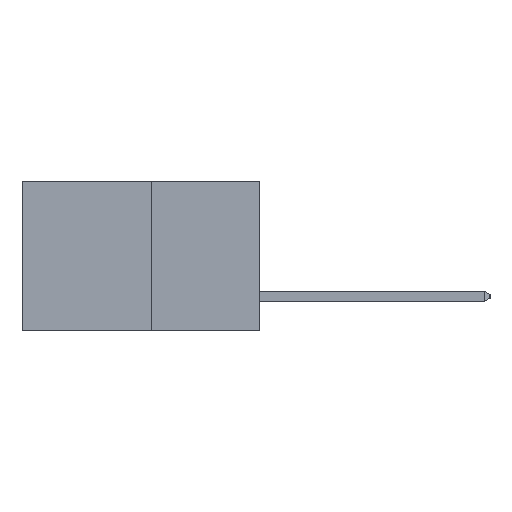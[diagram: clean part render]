
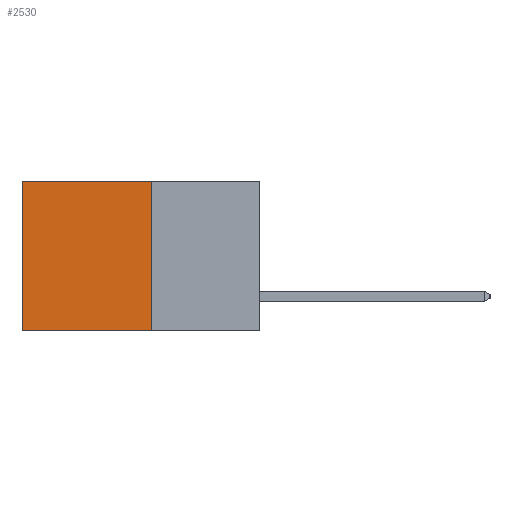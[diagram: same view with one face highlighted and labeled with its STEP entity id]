
A CAD part, left-side view. The second image highlights one B-rep face of the part: STEP entity #2530.
In plain terms, the highlighted planar face has unit normal (-1, 0, 0).
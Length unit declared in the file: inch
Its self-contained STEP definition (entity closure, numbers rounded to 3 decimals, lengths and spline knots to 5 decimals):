
#269 = EDGE_CURVE ( 'NONE', #4566, #11346, #6845, .T. ) ;
#826 = ORIENTED_EDGE ( 'NONE', *, *, #269, .T. ) ;
#2530 = ADVANCED_FACE ( 'NONE', ( #14349 ), #8832, .F. ) ;
#2600 = CARTESIAN_POINT ( 'NONE',  ( 0.277, 0.27, -0.37 ) ) ;
#3356 = EDGE_CURVE ( 'NONE', #13650, #11346, #5450, .T. ) ;
#4566 = VERTEX_POINT ( 'NONE', #12844 ) ;
#5028 = ORIENTED_EDGE ( 'NONE', *, *, #11836, .F. ) ;
#5037 = VECTOR ( 'NONE', #8416, 39.37008 ) ;
#5208 = DIRECTION ( 'NONE',  ( 0., 0., -1. ) ) ;
#5450 = LINE ( 'NONE', #8493, #5037 ) ;
#5720 = EDGE_CURVE ( 'NONE', #11275, #4566, #12967, .T. ) ;
#6845 = LINE ( 'NONE', #14623, #16168 ) ;
#8416 = DIRECTION ( 'NONE',  ( 0., 1., 0. ) ) ;
#8447 = DIRECTION ( 'NONE',  ( 0., 0., -1. ) ) ;
#8493 = CARTESIAN_POINT ( 'NONE',  ( 0.277, 0.27, -0.37 ) ) ;
#8512 = DIRECTION ( 'NONE',  ( 1., 0., 0. ) ) ;
#8688 = CARTESIAN_POINT ( 'NONE',  ( 0.277, 0.27, -0.37 ) ) ;
#8832 = PLANE ( 'NONE',  #9516 ) ;
#9516 = AXIS2_PLACEMENT_3D ( 'NONE', #8688, #8512, #8447 ) ;
#10386 = EDGE_LOOP ( 'NONE', ( #826, #14156, #5028, #14868 ) ) ;
#11191 = CARTESIAN_POINT ( 'NONE',  ( 0.277, 0.59, -0.37 ) ) ;
#11275 = VERTEX_POINT ( 'NONE', #13494 ) ;
#11346 = VERTEX_POINT ( 'NONE', #11191 ) ;
#11427 = CARTESIAN_POINT ( 'NONE',  ( 0.277, 0.27, -0.37 ) ) ;
#11446 = CARTESIAN_POINT ( 'NONE',  ( 0.277, 0.27, 0. ) ) ;
#11836 = EDGE_CURVE ( 'NONE', #11275, #13650, #15538, .T. ) ;
#11995 = VECTOR ( 'NONE', #5208, 39.37008 ) ;
#12741 = DIRECTION ( 'NONE',  ( 0., 1., 0. ) ) ;
#12844 = CARTESIAN_POINT ( 'NONE',  ( 0.277, 0.59, 0. ) ) ;
#12967 = LINE ( 'NONE', #11446, #15748 ) ;
#13494 = CARTESIAN_POINT ( 'NONE',  ( 0.277, 0.27, 0. ) ) ;
#13650 = VERTEX_POINT ( 'NONE', #2600 ) ;
#14156 = ORIENTED_EDGE ( 'NONE', *, *, #3356, .F. ) ;
#14349 = FACE_OUTER_BOUND ( 'NONE', #10386, .T. ) ;
#14503 = DIRECTION ( 'NONE',  ( 0., 0., -1. ) ) ;
#14623 = CARTESIAN_POINT ( 'NONE',  ( 0.277, 0.59, -0.37 ) ) ;
#14868 = ORIENTED_EDGE ( 'NONE', *, *, #5720, .T. ) ;
#15538 = LINE ( 'NONE', #11427, #11995 ) ;
#15748 = VECTOR ( 'NONE', #12741, 39.37008 ) ;
#16168 = VECTOR ( 'NONE', #14503, 39.37008 ) ;
